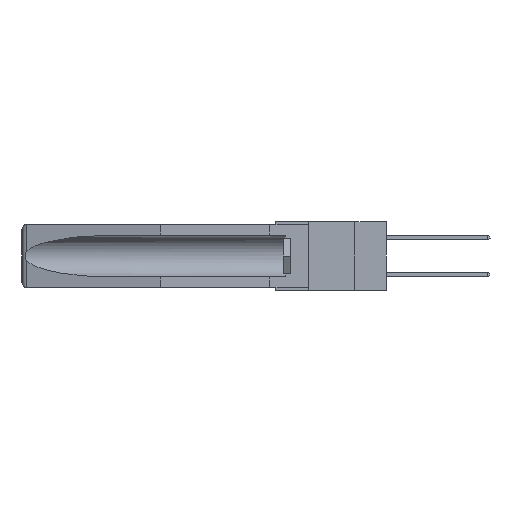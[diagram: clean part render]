
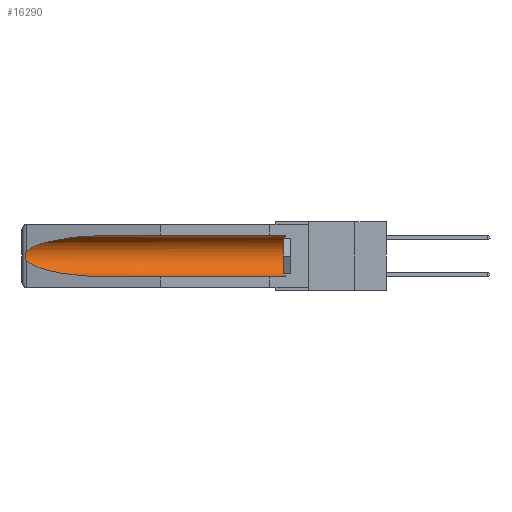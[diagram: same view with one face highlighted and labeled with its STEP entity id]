
A CAD part, left-side view. The second image highlights one B-rep face of the part: STEP entity #16290.
In plain terms, the highlighted cylindrical face has radius 2.857 mm (diameter 5.715 mm), a partial arc.
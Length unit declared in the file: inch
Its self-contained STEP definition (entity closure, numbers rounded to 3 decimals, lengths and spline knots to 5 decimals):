
#56 = VERTEX_POINT ( 'NONE', #520 ) ;
#203 = CARTESIAN_POINT ( 'NONE',  ( 0.2673, 1.53269, -0.17917 ) ) ;
#215 = EDGE_CURVE ( 'NONE', #18170, #5874, #2114, .T. ) ;
#217 = CARTESIAN_POINT ( 'NONE',  ( 0.155, 0.126, -0.1715 ) ) ;
#279 = CARTESIAN_POINT ( 'NONE',  ( 0.26537, 1.52718, -0.19328 ) ) ;
#520 = CARTESIAN_POINT ( 'NONE',  ( 0.155, 1.07973, -0.059 ) ) ;
#1538 = CARTESIAN_POINT ( 'NONE',  ( 0.26537, 1.52718, -0.14972 ) ) ;
#1546 = CARTESIAN_POINT ( 'NONE',  ( 0.155, -0.30754, -0.059 ) ) ;
#1673 = LINE ( 'NONE', #8668, #3395 ) ;
#2114 =( BOUNDED_CURVE ( )  B_SPLINE_CURVE ( 3, ( #17514, #19053, #11663, #11536 ),
 .UNSPECIFIED., .F., .F. ) 
 B_SPLINE_CURVE_WITH_KNOTS ( ( 4, 4 ),
 ( 0.1948, 1.5708 ),
 .UNSPECIFIED. ) 
 CURVE ( )  GEOMETRIC_REPRESENTATION_ITEM ( )  RATIONAL_B_SPLINE_CURVE ( ( 1., 0.848, 0.848, 1. ) ) 
 REPRESENTATION_ITEM ( '' )  );
#2400 = CARTESIAN_POINT ( 'NONE',  ( 0.155, 0.126, -0.284 ) ) ;
#2401 = ORIENTED_EDGE ( 'NONE', *, *, #11101, .T. ) ;
#2778 =( BOUNDED_CURVE ( )  B_SPLINE_CURVE ( 3, ( #12640, #5171, #17148, #17276 ),
 .UNSPECIFIED., .F., .F. ) 
 B_SPLINE_CURVE_WITH_KNOTS ( ( 4, 4 ),
 ( 4.71239, 6.08839 ),
 .UNSPECIFIED. ) 
 CURVE ( )  GEOMETRIC_REPRESENTATION_ITEM ( )  RATIONAL_B_SPLINE_CURVE ( ( 1., 0.848, 0.848, 1. ) ) 
 REPRESENTATION_ITEM ( '' )  );
#3137 = DIRECTION ( 'NONE',  ( 0., 1., 0. ) ) ;
#3374 = CARTESIAN_POINT ( 'NONE',  ( 0.26655, 1.53094, -0.18657 ) ) ;
#3395 = VECTOR ( 'NONE', #19367, 39.37008 ) ;
#3433 = ORIENTED_EDGE ( 'NONE', *, *, #11862, .T. ) ;
#3519 = DIRECTION ( 'NONE',  ( 0., -1., 0. ) ) ;
#4487 = VERTEX_POINT ( 'NONE', #1538 ) ;
#4727 = VERTEX_POINT ( 'NONE', #12678 ) ;
#4735 = ORIENTED_EDGE ( 'NONE', *, *, #215, .T. ) ;
#4833 = CARTESIAN_POINT ( 'NONE',  ( 0.26654, 1.53092, -0.15636 ) ) ;
#4884 = CYLINDRICAL_SURFACE ( 'NONE', #5825, 0.1125 ) ;
#4906 = CARTESIAN_POINT ( 'NONE',  ( 0.26597, 1.5296, -0.19026 ) ) ;
#5115 = FACE_OUTER_BOUND ( 'NONE', #7939, .T. ) ;
#5171 = CARTESIAN_POINT ( 'NONE',  ( 0.21114, 1.30732, -0.059 ) ) ;
#5825 = AXIS2_PLACEMENT_3D ( 'NONE', #13480, #7621, #11978 ) ;
#5874 = VERTEX_POINT ( 'NONE', #13492 ) ;
#6383 = CARTESIAN_POINT ( 'NONE',  ( 0.2675, 1.53308, -0.16763 ) ) ;
#7026 = CARTESIAN_POINT ( 'NONE',  ( 0.26537, 1.52718, -0.19328 ) ) ;
#7396 = EDGE_CURVE ( 'NONE', #4487, #18170, #18214, .T. ) ;
#7621 = DIRECTION ( 'NONE',  ( 0., 1., 0. ) ) ;
#7840 = CARTESIAN_POINT ( 'NONE',  ( 0.26537, 1.52718, -0.14972 ) ) ;
#7909 = CARTESIAN_POINT ( 'NONE',  ( 0.2673, 1.5327, -0.16383 ) ) ;
#7939 = EDGE_LOOP ( 'NONE', ( #2401, #17158, #4735, #17100, #3433, #18788 ) ) ;
#8668 = CARTESIAN_POINT ( 'NONE',  ( 0.155, -0.30754, -0.284 ) ) ;
#8911 = EDGE_CURVE ( 'NONE', #4727, #56, #10415, .T. ) ;
#10305 = AXIS2_PLACEMENT_3D ( 'NONE', #217, #3519, #10892 ) ;
#10415 = LINE ( 'NONE', #1546, #11834 ) ;
#10892 = DIRECTION ( 'NONE',  ( 0., 0., 1. ) ) ;
#11101 = EDGE_CURVE ( 'NONE', #56, #4487, #2778, .T. ) ;
#11514 = CIRCLE ( 'NONE', #10305, 0.1125 ) ;
#11536 = CARTESIAN_POINT ( 'NONE',  ( 0.155, 1.07973, -0.284 ) ) ;
#11663 = CARTESIAN_POINT ( 'NONE',  ( 0.21114, 1.30732, -0.284 ) ) ;
#11834 = VECTOR ( 'NONE', #3137, 39.37008 ) ;
#11862 = EDGE_CURVE ( 'NONE', #14261, #4727, #11514, .T. ) ;
#11978 = DIRECTION ( 'NONE',  ( 0., 0., 1. ) ) ;
#12640 = CARTESIAN_POINT ( 'NONE',  ( 0.155, 1.07973, -0.059 ) ) ;
#12678 = CARTESIAN_POINT ( 'NONE',  ( 0.155, 0.126, -0.059 ) ) ;
#13480 = CARTESIAN_POINT ( 'NONE',  ( 0.155, -0.30754, -0.1715 ) ) ;
#13492 = CARTESIAN_POINT ( 'NONE',  ( 0.155, 1.07973, -0.284 ) ) ;
#14261 = VERTEX_POINT ( 'NONE', #2400 ) ;
#16290 = ADVANCED_FACE ( 'NONE', ( #5115 ), #4884, .F. ) ;
#17100 = ORIENTED_EDGE ( 'NONE', *, *, #17362, .F. ) ;
#17148 = CARTESIAN_POINT ( 'NONE',  ( 0.25451, 1.48313, -0.09465 ) ) ;
#17158 = ORIENTED_EDGE ( 'NONE', *, *, #7396, .T. ) ;
#17276 = CARTESIAN_POINT ( 'NONE',  ( 0.26537, 1.52718, -0.14972 ) ) ;
#17362 = EDGE_CURVE ( 'NONE', #14261, #5874, #1673, .T. ) ;
#17514 = CARTESIAN_POINT ( 'NONE',  ( 0.26537, 1.52718, -0.19328 ) ) ;
#18170 = VERTEX_POINT ( 'NONE', #7026 ) ;
#18214 = B_SPLINE_CURVE_WITH_KNOTS ( 'NONE', 3,
 ( #7840, #18449, #4833, #7909, #6383, #18379, #203, #3374, #4906, #279 ),
 .UNSPECIFIED., .F., .F.,
 ( 4, 2, 2, 2, 4 ),
 ( 0., 0.00029, 0.00058, 0.00087, 0.00117 ),
 .UNSPECIFIED. ) ;
#18379 = CARTESIAN_POINT ( 'NONE',  ( 0.2675, 1.53308, -0.17534 ) ) ;
#18449 = CARTESIAN_POINT ( 'NONE',  ( 0.26597, 1.52961, -0.15275 ) ) ;
#18788 = ORIENTED_EDGE ( 'NONE', *, *, #8911, .T. ) ;
#19053 = CARTESIAN_POINT ( 'NONE',  ( 0.25451, 1.48313, -0.24835 ) ) ;
#19367 = DIRECTION ( 'NONE',  ( 0., 1., 0. ) ) ;
